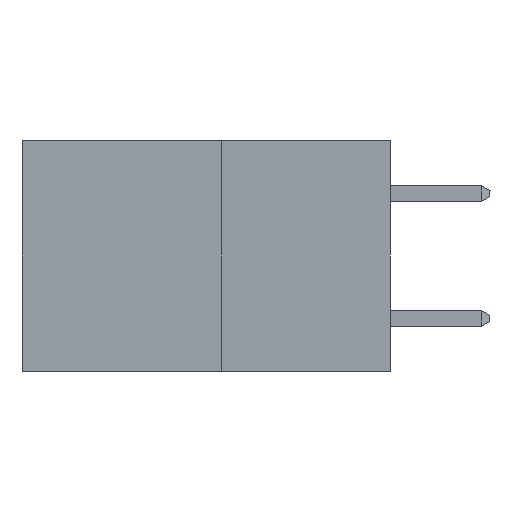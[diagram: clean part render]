
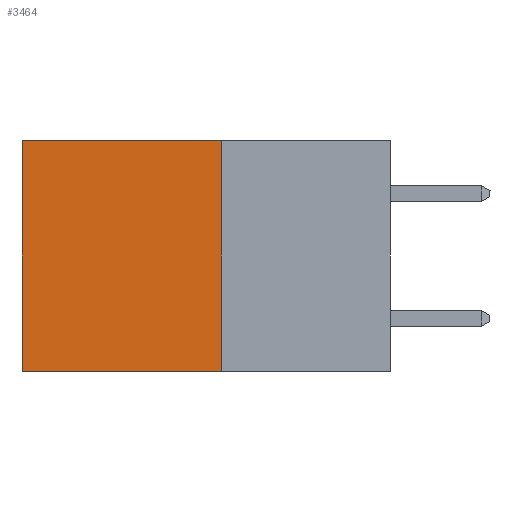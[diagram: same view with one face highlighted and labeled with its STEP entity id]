
A CAD part, left-side view. The second image highlights one B-rep face of the part: STEP entity #3464.
In plain terms, the highlighted planar face has unit normal (-1, 0, 0).
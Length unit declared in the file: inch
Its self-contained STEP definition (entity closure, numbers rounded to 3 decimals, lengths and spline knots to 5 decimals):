
#554 = EDGE_CURVE ( 'NONE', #18040, #3389, #5741, .T. ) ;
#579 = CARTESIAN_POINT ( 'NONE',  ( 0.277, 0.27, -0.37 ) ) ;
#638 = DIRECTION ( 'NONE',  ( 0., 0., -1. ) ) ;
#958 = ORIENTED_EDGE ( 'NONE', *, *, #7656, .T. ) ;
#1180 = CARTESIAN_POINT ( 'NONE',  ( 0.277, 0.27, -0.37 ) ) ;
#2317 = VECTOR ( 'NONE', #10331, 39.37008 ) ;
#2395 = CARTESIAN_POINT ( 'NONE',  ( 0.277, 0.59, -0.37 ) ) ;
#3192 = DIRECTION ( 'NONE',  ( 0., 1., 0. ) ) ;
#3389 = VERTEX_POINT ( 'NONE', #8094 ) ;
#3464 = ADVANCED_FACE ( 'NONE', ( #5663 ), #6698, .F. ) ;
#3646 = ORIENTED_EDGE ( 'NONE', *, *, #17278, .F. ) ;
#4786 = VECTOR ( 'NONE', #19113, 39.37008 ) ;
#5079 = CARTESIAN_POINT ( 'NONE',  ( 0.277, 0.27, 0. ) ) ;
#5663 = FACE_OUTER_BOUND ( 'NONE', #14077, .T. ) ;
#5741 = LINE ( 'NONE', #2395, #4786 ) ;
#6343 = LINE ( 'NONE', #1180, #2317 ) ;
#6516 = VERTEX_POINT ( 'NONE', #5079 ) ;
#6698 = PLANE ( 'NONE',  #8234 ) ;
#7013 = VECTOR ( 'NONE', #7527, 39.37008 ) ;
#7527 = DIRECTION ( 'NONE',  ( 0., 0., -1. ) ) ;
#7656 = EDGE_CURVE ( 'NONE', #6516, #18040, #9059, .T. ) ;
#7870 = VERTEX_POINT ( 'NONE', #17436 ) ;
#8094 = CARTESIAN_POINT ( 'NONE',  ( 0.277, 0.59, -0.37 ) ) ;
#8231 = CARTESIAN_POINT ( 'NONE',  ( 0.277, 0.59, 0. ) ) ;
#8234 = AXIS2_PLACEMENT_3D ( 'NONE', #579, #9777, #638 ) ;
#9059 = LINE ( 'NONE', #13880, #12639 ) ;
#9777 = DIRECTION ( 'NONE',  ( 1., 0., 0. ) ) ;
#10331 = DIRECTION ( 'NONE',  ( 0., 1., 0. ) ) ;
#10556 = EDGE_CURVE ( 'NONE', #6516, #7870, #10615, .T. ) ;
#10615 = LINE ( 'NONE', #16681, #7013 ) ;
#12639 = VECTOR ( 'NONE', #3192, 39.37008 ) ;
#13106 = ORIENTED_EDGE ( 'NONE', *, *, #10556, .F. ) ;
#13880 = CARTESIAN_POINT ( 'NONE',  ( 0.277, 0.27, 0. ) ) ;
#14077 = EDGE_LOOP ( 'NONE', ( #14939, #3646, #13106, #958 ) ) ;
#14939 = ORIENTED_EDGE ( 'NONE', *, *, #554, .T. ) ;
#16681 = CARTESIAN_POINT ( 'NONE',  ( 0.277, 0.27, -0.37 ) ) ;
#17278 = EDGE_CURVE ( 'NONE', #7870, #3389, #6343, .T. ) ;
#17436 = CARTESIAN_POINT ( 'NONE',  ( 0.277, 0.27, -0.37 ) ) ;
#18040 = VERTEX_POINT ( 'NONE', #8231 ) ;
#19113 = DIRECTION ( 'NONE',  ( 0., 0., -1. ) ) ;
